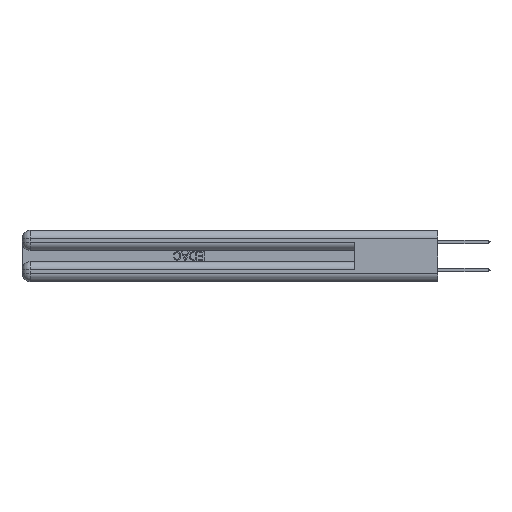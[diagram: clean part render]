
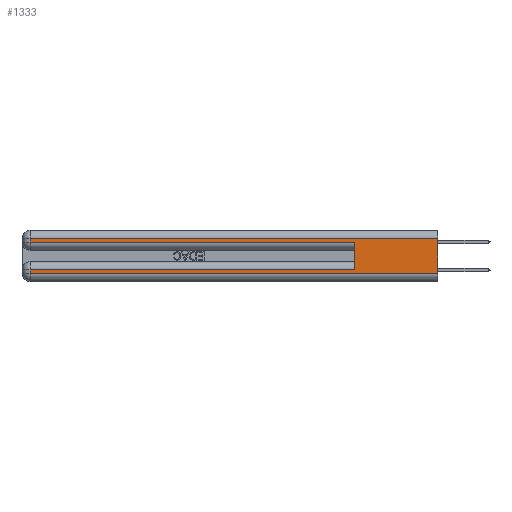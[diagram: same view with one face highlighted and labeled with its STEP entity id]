
A CAD part, left-side view. The second image highlights one B-rep face of the part: STEP entity #1333.
In plain terms, the highlighted planar face has unit normal (-1, 0, 0).
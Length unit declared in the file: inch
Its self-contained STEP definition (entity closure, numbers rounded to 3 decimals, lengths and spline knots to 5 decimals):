
#326 = EDGE_CURVE ( 'NONE', #49297, #41463, #10787, .T. ) ;
#695 = CARTESIAN_POINT ( 'NONE',  ( 0., 0., 0.06 ) ) ;
#1333 = ADVANCED_FACE ( 'NONE', ( #4521 ), #30881, .F. ) ;
#1833 = LINE ( 'NONE', #41169, #4893 ) ;
#1936 = DIRECTION ( 'NONE',  ( 0., 0., 1. ) ) ;
#2367 = DIRECTION ( 'NONE',  ( 0., 0., -1. ) ) ;
#4306 = EDGE_CURVE ( 'NONE', #49297, #23448, #1833, .T. ) ;
#4443 = VECTOR ( 'NONE', #28532, 39.37008 ) ;
#4521 = FACE_OUTER_BOUND ( 'NONE', #50148, .T. ) ;
#4893 = VECTOR ( 'NONE', #1936, 39.37008 ) ;
#5645 = VECTOR ( 'NONE', #44209, 39.37008 ) ;
#5691 = VECTOR ( 'NONE', #2367, 39.37008 ) ;
#6094 = CARTESIAN_POINT ( 'NONE',  ( 0., 2.94, 0.285 ) ) ;
#6390 = VERTEX_POINT ( 'NONE', #32508 ) ;
#6829 = LINE ( 'NONE', #32498, #50667 ) ;
#7199 = DIRECTION ( 'NONE',  ( 1., 0., 0. ) ) ;
#7490 = LINE ( 'NONE', #48410, #22929 ) ;
#7798 = CARTESIAN_POINT ( 'NONE',  ( 0., 0.6, 0.285 ) ) ;
#8044 = CARTESIAN_POINT ( 'NONE',  ( 0., 2.94, 0.31 ) ) ;
#8451 = CARTESIAN_POINT ( 'NONE',  ( 0., 0., 0.285 ) ) ;
#8684 = CARTESIAN_POINT ( 'NONE',  ( 0., 2.94, 0.085 ) ) ;
#9009 = CARTESIAN_POINT ( 'NONE',  ( 0., 0., 0.37 ) ) ;
#10787 = LINE ( 'NONE', #33783, #38646 ) ;
#11224 = ORIENTED_EDGE ( 'NONE', *, *, #41628, .F. ) ;
#13683 = LINE ( 'NONE', #49526, #5691 ) ;
#13787 = EDGE_CURVE ( 'NONE', #41463, #6390, #7490, .T. ) ;
#14357 = VERTEX_POINT ( 'NONE', #35724 ) ;
#14571 = ORIENTED_EDGE ( 'NONE', *, *, #326, .T. ) ;
#17299 = ORIENTED_EDGE ( 'NONE', *, *, #23006, .T. ) ;
#18070 = DIRECTION ( 'NONE',  ( 0., 1., 0. ) ) ;
#20591 = VERTEX_POINT ( 'NONE', #6094 ) ;
#22929 = VECTOR ( 'NONE', #25228, 39.37008 ) ;
#23006 = EDGE_CURVE ( 'NONE', #6390, #34380, #39213, .T. ) ;
#23448 = VERTEX_POINT ( 'NONE', #7798 ) ;
#25052 = DIRECTION ( 'NONE',  ( 0., 1., 0. ) ) ;
#25228 = DIRECTION ( 'NONE',  ( 0., 0., -1. ) ) ;
#26361 = CARTESIAN_POINT ( 'NONE',  ( 0., 0., 0.37 ) ) ;
#27421 = ORIENTED_EDGE ( 'NONE', *, *, #34483, .T. ) ;
#28532 = DIRECTION ( 'NONE',  ( 0., 0., -1. ) ) ;
#29838 = CARTESIAN_POINT ( 'NONE',  ( 0., 0.6, 0.085 ) ) ;
#30425 = LINE ( 'NONE', #9009, #4443 ) ;
#30881 = PLANE ( 'NONE',  #35015 ) ;
#32498 = CARTESIAN_POINT ( 'NONE',  ( 0., 0., 0.31 ) ) ;
#32508 = CARTESIAN_POINT ( 'NONE',  ( 0., 2.94, 0.06 ) ) ;
#33241 = CARTESIAN_POINT ( 'NONE',  ( 0., 0., 0.06 ) ) ;
#33783 = CARTESIAN_POINT ( 'NONE',  ( 0., 0., 0.085 ) ) ;
#34380 = VERTEX_POINT ( 'NONE', #695 ) ;
#34483 = EDGE_CURVE ( 'NONE', #20591, #23448, #43930, .T. ) ;
#35015 = AXIS2_PLACEMENT_3D ( 'NONE', #26361, #7199, #37968 ) ;
#35724 = CARTESIAN_POINT ( 'NONE',  ( 0., 0., 0.31 ) ) ;
#35997 = ORIENTED_EDGE ( 'NONE', *, *, #49267, .T. ) ;
#36086 = VECTOR ( 'NONE', #36884, 39.37008 ) ;
#36884 = DIRECTION ( 'NONE',  ( 0., -1., 0. ) ) ;
#37968 = DIRECTION ( 'NONE',  ( 0., 0., -1. ) ) ;
#38327 = ORIENTED_EDGE ( 'NONE', *, *, #13787, .T. ) ;
#38646 = VECTOR ( 'NONE', #18070, 39.37008 ) ;
#39213 = LINE ( 'NONE', #33241, #36086 ) ;
#40259 = ORIENTED_EDGE ( 'NONE', *, *, #42795, .T. ) ;
#40600 = ORIENTED_EDGE ( 'NONE', *, *, #4306, .F. ) ;
#41169 = CARTESIAN_POINT ( 'NONE',  ( 0., 0.6, 0.145 ) ) ;
#41463 = VERTEX_POINT ( 'NONE', #8684 ) ;
#41628 = EDGE_CURVE ( 'NONE', #14357, #34380, #30425, .T. ) ;
#42795 = EDGE_CURVE ( 'NONE', #14357, #49374, #6829, .T. ) ;
#43930 = LINE ( 'NONE', #8451, #5645 ) ;
#44209 = DIRECTION ( 'NONE',  ( 0., -1., 0. ) ) ;
#48410 = CARTESIAN_POINT ( 'NONE',  ( 0., 2.94, 0.37 ) ) ;
#49267 = EDGE_CURVE ( 'NONE', #49374, #20591, #13683, .T. ) ;
#49297 = VERTEX_POINT ( 'NONE', #29838 ) ;
#49374 = VERTEX_POINT ( 'NONE', #8044 ) ;
#49526 = CARTESIAN_POINT ( 'NONE',  ( 0., 2.94, 0.37 ) ) ;
#50148 = EDGE_LOOP ( 'NONE', ( #11224, #40259, #35997, #27421, #40600, #14571, #38327, #17299 ) ) ;
#50667 = VECTOR ( 'NONE', #25052, 39.37008 ) ;
